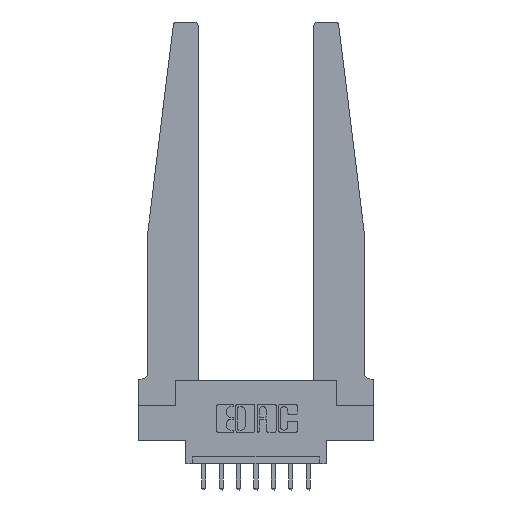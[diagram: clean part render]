
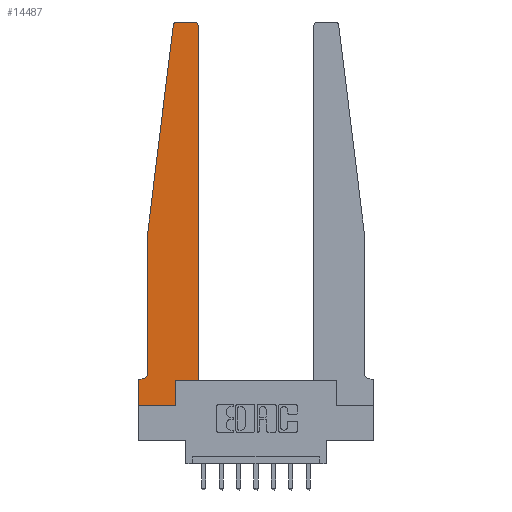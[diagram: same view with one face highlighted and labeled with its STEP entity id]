
A CAD part, top view. The second image highlights one B-rep face of the part: STEP entity #14487.
In plain terms, the highlighted planar face has unit normal (0, 0, 1).
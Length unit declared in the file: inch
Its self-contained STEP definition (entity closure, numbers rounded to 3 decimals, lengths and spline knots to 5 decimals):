
#291 = DIRECTION ( 'NONE',  ( 0., -1., 0. ) ) ;
#507 = LINE ( 'NONE', #10586, #8790 ) ;
#646 = AXIS2_PLACEMENT_3D ( 'NONE', #9924, #5447, #4498 ) ;
#994 = LINE ( 'NONE', #11359, #5048 ) ;
#1014 = ORIENTED_EDGE ( 'NONE', *, *, #6273, .T. ) ;
#1088 = LINE ( 'NONE', #10000, #7497 ) ;
#1174 = DIRECTION ( 'NONE',  ( 1., 0., 0. ) ) ;
#1378 = LINE ( 'NONE', #10369, #12935 ) ;
#1568 = EDGE_CURVE ( 'NONE', #9244, #13920, #6169, .T. ) ;
#1590 = CARTESIAN_POINT ( 'NONE',  ( 0.25, 2.75, 0.37 ) ) ;
#1672 = CARTESIAN_POINT ( 'NONE',  ( 0.425, 0.18, 0.37 ) ) ;
#1791 = VERTEX_POINT ( 'NONE', #13267 ) ;
#2209 = CIRCLE ( 'NONE', #10441, 0.05 ) ;
#2269 = DIRECTION ( 'NONE',  ( -1., 0., 0. ) ) ;
#2362 = LINE ( 'NONE', #9214, #13310 ) ;
#2413 = CARTESIAN_POINT ( 'NONE',  ( 0.015, 0.2375, 0.37 ) ) ;
#3527 = CARTESIAN_POINT ( 'NONE',  ( 0.2605, 0., 0.37 ) ) ;
#3622 = DIRECTION ( 'NONE',  ( 0., 1., 0. ) ) ;
#4081 = CARTESIAN_POINT ( 'NONE',  ( 0.27653, 2.72, 0.37 ) ) ;
#4149 = LINE ( 'NONE', #9727, #10124 ) ;
#4498 = DIRECTION ( 'NONE',  ( 1., 0., 0. ) ) ;
#4515 = AXIS2_PLACEMENT_3D ( 'NONE', #4081, #9945, #8556 ) ;
#4691 = DIRECTION ( 'NONE',  ( 0., -1., 0. ) ) ;
#4754 = AXIS2_PLACEMENT_3D ( 'NONE', #7756, #13540, #10203 ) ;
#5048 = VECTOR ( 'NONE', #4691, 39.37008 ) ;
#5109 = CARTESIAN_POINT ( 'NONE',  ( 0.065, 0.2375, 0.37 ) ) ;
#5236 = ORIENTED_EDGE ( 'NONE', *, *, #12591, .T. ) ;
#5447 = DIRECTION ( 'NONE',  ( 0., 0., 1. ) ) ;
#5710 = LINE ( 'NONE', #9103, #8543 ) ;
#5799 = EDGE_LOOP ( 'NONE', ( #9593, #12570, #7050, #12449, #8394, #7975, #10050, #1014, #9629, #12581, #5236, #6831 ) ) ;
#6169 = LINE ( 'NONE', #1590, #13349 ) ;
#6242 = DIRECTION ( 'NONE',  ( -1., 0., 0. ) ) ;
#6273 = EDGE_CURVE ( 'NONE', #14309, #11889, #507, .T. ) ;
#6296 = VERTEX_POINT ( 'NONE', #1672 ) ;
#6338 = CARTESIAN_POINT ( 'NONE',  ( 0., 0.1875, 0.37 ) ) ;
#6640 = EDGE_CURVE ( 'NONE', #6812, #13122, #2209, .T. ) ;
#6812 = VERTEX_POINT ( 'NONE', #5109 ) ;
#6831 = ORIENTED_EDGE ( 'NONE', *, *, #8813, .T. ) ;
#6904 = VERTEX_POINT ( 'NONE', #12358 ) ;
#6972 = PLANE ( 'NONE',  #4754 ) ;
#7050 = ORIENTED_EDGE ( 'NONE', *, *, #7560, .T. ) ;
#7188 = CARTESIAN_POINT ( 'NONE',  ( 0.425, 2.72, 0.37 ) ) ;
#7258 = EDGE_CURVE ( 'NONE', #6904, #6296, #2362, .T. ) ;
#7497 = VECTOR ( 'NONE', #12035, 39.37008 ) ;
#7560 = EDGE_CURVE ( 'NONE', #1791, #13293, #1088, .T. ) ;
#7756 = CARTESIAN_POINT ( 'NONE',  ( 0., 0.1875, 0.37 ) ) ;
#7854 = DIRECTION ( 'NONE',  ( 0., 0., -1. ) ) ;
#7975 = ORIENTED_EDGE ( 'NONE', *, *, #9322, .T. ) ;
#8277 = CARTESIAN_POINT ( 'NONE',  ( 0., 0., 0.37 ) ) ;
#8394 = ORIENTED_EDGE ( 'NONE', *, *, #6640, .T. ) ;
#8543 = VECTOR ( 'NONE', #13542, 39.37008 ) ;
#8556 = DIRECTION ( 'NONE',  ( 1., 0., 0. ) ) ;
#8636 = CIRCLE ( 'NONE', #646, 0.03 ) ;
#8790 = VECTOR ( 'NONE', #12771, 39.37008 ) ;
#8813 = EDGE_CURVE ( 'NONE', #9496, #9244, #8636, .T. ) ;
#9028 = FACE_OUTER_BOUND ( 'NONE', #5799, .T. ) ;
#9103 = CARTESIAN_POINT ( 'NONE',  ( 0.065, 0.1875, 0.37 ) ) ;
#9214 = CARTESIAN_POINT ( 'NONE',  ( 0.425, 0.18, 0.37 ) ) ;
#9244 = VERTEX_POINT ( 'NONE', #13264 ) ;
#9289 = EDGE_CURVE ( 'NONE', #13503, #14309, #994, .T. ) ;
#9322 = EDGE_CURVE ( 'NONE', #13122, #13503, #5710, .T. ) ;
#9496 = VERTEX_POINT ( 'NONE', #7188 ) ;
#9553 = CARTESIAN_POINT ( 'NONE',  ( 0.27653, 2.75, 0.37 ) ) ;
#9593 = ORIENTED_EDGE ( 'NONE', *, *, #1568, .T. ) ;
#9629 = ORIENTED_EDGE ( 'NONE', *, *, #11146, .T. ) ;
#9727 = CARTESIAN_POINT ( 'NONE',  ( 0.2605, 0.18, 0.37 ) ) ;
#9904 = CIRCLE ( 'NONE', #4515, 0.03 ) ;
#9924 = CARTESIAN_POINT ( 'NONE',  ( 0.395, 2.72, 0.37 ) ) ;
#9945 = DIRECTION ( 'NONE',  ( 0., 0., 1. ) ) ;
#10000 = CARTESIAN_POINT ( 'NONE',  ( 0.065, 1.25, 0.37 ) ) ;
#10050 = ORIENTED_EDGE ( 'NONE', *, *, #9289, .T. ) ;
#10124 = VECTOR ( 'NONE', #14102, 39.37008 ) ;
#10203 = DIRECTION ( 'NONE',  ( 1., 0., 0. ) ) ;
#10369 = CARTESIAN_POINT ( 'NONE',  ( 0.065, 1.25, 0.37 ) ) ;
#10441 = AXIS2_PLACEMENT_3D ( 'NONE', #2413, #7854, #2269 ) ;
#10522 = CARTESIAN_POINT ( 'NONE',  ( 0.425, 0.18, 0.37 ) ) ;
#10586 = CARTESIAN_POINT ( 'NONE',  ( 0., 0., 0.37 ) ) ;
#11146 = EDGE_CURVE ( 'NONE', #11889, #6904, #4149, .T. ) ;
#11342 = CARTESIAN_POINT ( 'NONE',  ( 0.065, 1.25, 0.37 ) ) ;
#11359 = CARTESIAN_POINT ( 'NONE',  ( 0., 0., 0.37 ) ) ;
#11889 = VERTEX_POINT ( 'NONE', #3527 ) ;
#12035 = DIRECTION ( 'NONE',  ( -0.122, -0.992, 0. ) ) ;
#12358 = CARTESIAN_POINT ( 'NONE',  ( 0.2605, 0.18, 0.37 ) ) ;
#12449 = ORIENTED_EDGE ( 'NONE', *, *, #12929, .T. ) ;
#12471 = EDGE_CURVE ( 'NONE', #13920, #1791, #9904, .T. ) ;
#12570 = ORIENTED_EDGE ( 'NONE', *, *, #12471, .T. ) ;
#12581 = ORIENTED_EDGE ( 'NONE', *, *, #7258, .T. ) ;
#12591 = EDGE_CURVE ( 'NONE', #6296, #9496, #13509, .T. ) ;
#12771 = DIRECTION ( 'NONE',  ( 1., 0., 0. ) ) ;
#12801 = CARTESIAN_POINT ( 'NONE',  ( 0.015, 0.1875, 0.37 ) ) ;
#12929 = EDGE_CURVE ( 'NONE', #13293, #6812, #1378, .T. ) ;
#12935 = VECTOR ( 'NONE', #291, 39.37008 ) ;
#13122 = VERTEX_POINT ( 'NONE', #12801 ) ;
#13264 = CARTESIAN_POINT ( 'NONE',  ( 0.395, 2.75, 0.37 ) ) ;
#13267 = CARTESIAN_POINT ( 'NONE',  ( 0.24675, 2.72367, 0.37 ) ) ;
#13293 = VERTEX_POINT ( 'NONE', #11342 ) ;
#13310 = VECTOR ( 'NONE', #1174, 39.37008 ) ;
#13349 = VECTOR ( 'NONE', #6242, 39.37008 ) ;
#13503 = VERTEX_POINT ( 'NONE', #6338 ) ;
#13509 = LINE ( 'NONE', #10522, #13855 ) ;
#13540 = DIRECTION ( 'NONE',  ( 0., 0., 1. ) ) ;
#13542 = DIRECTION ( 'NONE',  ( -1., 0., 0. ) ) ;
#13855 = VECTOR ( 'NONE', #3622, 39.37008 ) ;
#13920 = VERTEX_POINT ( 'NONE', #9553 ) ;
#14102 = DIRECTION ( 'NONE',  ( 0., 1., 0. ) ) ;
#14309 = VERTEX_POINT ( 'NONE', #8277 ) ;
#14487 = ADVANCED_FACE ( 'NONE', ( #9028 ), #6972, .T. ) ;
